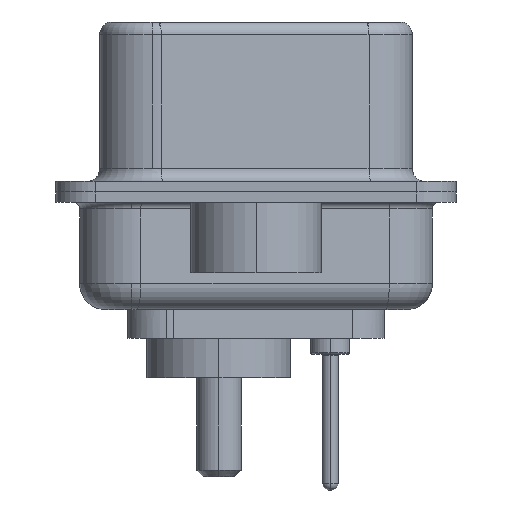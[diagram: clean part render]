
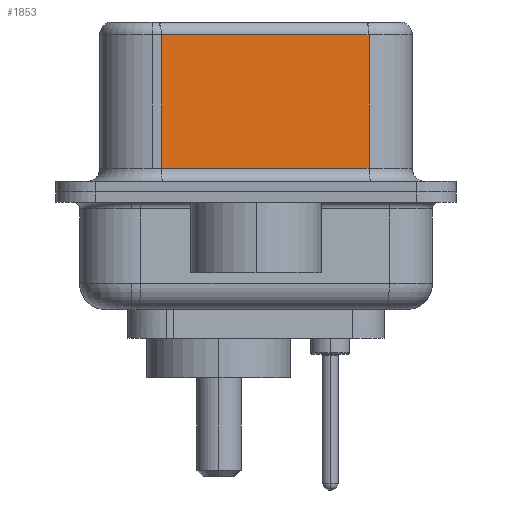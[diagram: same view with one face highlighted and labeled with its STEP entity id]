
A CAD part, left-side view. The second image highlights one B-rep face of the part: STEP entity #1853.
In plain terms, the highlighted planar face has unit normal (-0.985, -0.174, 0).
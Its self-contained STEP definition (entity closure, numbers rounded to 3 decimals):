
#282 = VERTEX_POINT ( 'NONE', #4873 ) ;
#872 = CARTESIAN_POINT ( 'NONE',  ( 3.73, 3.628, 6.52 ) ) ;
#1046 = PLANE ( 'NONE',  #1348 ) ;
#1276 = VECTOR ( 'NONE', #18780, 1000. ) ;
#1348 = AXIS2_PLACEMENT_3D ( 'NONE', #2949, #4721, #4569 ) ;
#1853 = ADVANCED_FACE ( 'NONE', ( #5039 ), #1046, .F. ) ;
#2949 = CARTESIAN_POINT ( 'NONE',  ( 5.132, -4.322, 6.52 ) ) ;
#3845 = CARTESIAN_POINT ( 'NONE',  ( 3.73, 3.628, 0.9 ) ) ;
#4569 = DIRECTION ( 'NONE',  ( -0.174, 0.985, 0. ) ) ;
#4721 = DIRECTION ( 'NONE',  ( 0.985, 0.174, 0. ) ) ;
#4753 = EDGE_CURVE ( 'NONE', #12175, #5321, #13733, .T. ) ;
#4873 = CARTESIAN_POINT ( 'NONE',  ( 5.132, -4.322, 6.02 ) ) ;
#5039 = FACE_OUTER_BOUND ( 'NONE', #12731, .T. ) ;
#5321 = VERTEX_POINT ( 'NONE', #3845 ) ;
#5627 = CARTESIAN_POINT ( 'NONE',  ( 5.132, -4.322, 6.52 ) ) ;
#7611 = DIRECTION ( 'NONE',  ( 0., 0., -1. ) ) ;
#8937 = CARTESIAN_POINT ( 'NONE',  ( 3.73, 3.628, 6.02 ) ) ;
#9626 = ORIENTED_EDGE ( 'NONE', *, *, #11723, .T. ) ;
#9645 = VECTOR ( 'NONE', #14490, 1000. ) ;
#10168 = LINE ( 'NONE', #16159, #9645 ) ;
#10665 = ORIENTED_EDGE ( 'NONE', *, *, #4753, .T. ) ;
#10978 = LINE ( 'NONE', #13253, #18748 ) ;
#11262 = ORIENTED_EDGE ( 'NONE', *, *, #12152, .F. ) ;
#11723 = EDGE_CURVE ( 'NONE', #282, #12175, #10168, .T. ) ;
#12152 = EDGE_CURVE ( 'NONE', #282, #21451, #18943, .T. ) ;
#12175 = VERTEX_POINT ( 'NONE', #8937 ) ;
#12731 = EDGE_LOOP ( 'NONE', ( #11262, #9626, #10665, #16571 ) ) ;
#13253 = CARTESIAN_POINT ( 'NONE',  ( 5.132, -4.322, 0.9 ) ) ;
#13733 = LINE ( 'NONE', #872, #17607 ) ;
#14490 = DIRECTION ( 'NONE',  ( -0.174, 0.985, 0. ) ) ;
#16159 = CARTESIAN_POINT ( 'NONE',  ( 5.132, -4.322, 6.02 ) ) ;
#16571 = ORIENTED_EDGE ( 'NONE', *, *, #20603, .T. ) ;
#16958 = CARTESIAN_POINT ( 'NONE',  ( 5.132, -4.322, 0.9 ) ) ;
#17607 = VECTOR ( 'NONE', #7611, 1000. ) ;
#18253 = DIRECTION ( 'NONE',  ( 0.174, -0.985, 0. ) ) ;
#18748 = VECTOR ( 'NONE', #18253, 1000. ) ;
#18780 = DIRECTION ( 'NONE',  ( 0., 0., -1. ) ) ;
#18943 = LINE ( 'NONE', #5627, #1276 ) ;
#20603 = EDGE_CURVE ( 'NONE', #5321, #21451, #10978, .T. ) ;
#21451 = VERTEX_POINT ( 'NONE', #16958 ) ;
